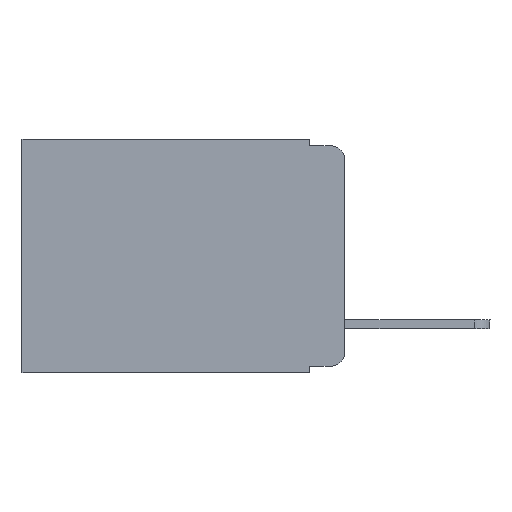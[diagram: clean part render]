
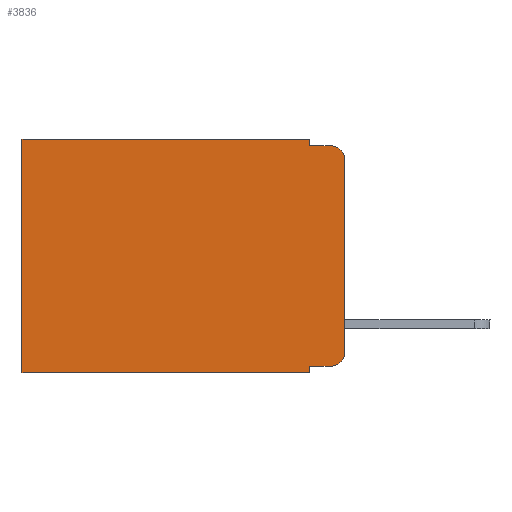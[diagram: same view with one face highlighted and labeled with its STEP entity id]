
A CAD part, left-side view. The second image highlights one B-rep face of the part: STEP entity #3836.
In plain terms, the highlighted planar face has unit normal (-1, 0, 0).
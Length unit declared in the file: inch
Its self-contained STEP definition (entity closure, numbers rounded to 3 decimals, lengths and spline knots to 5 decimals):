
#102 = CARTESIAN_POINT ( 'NONE',  ( 0.298, 0., 0. ) ) ;
#114 = DIRECTION ( 'NONE',  ( 0., 0., -1. ) ) ;
#173 = DIRECTION ( 'NONE',  ( -1., 0., 0. ) ) ;
#221 = VERTEX_POINT ( 'NONE', #9424 ) ;
#527 = ORIENTED_EDGE ( 'NONE', *, *, #11059, .T. ) ;
#671 = CARTESIAN_POINT ( 'NONE',  ( 0.298, 0.051, -0.01 ) ) ;
#741 = ORIENTED_EDGE ( 'NONE', *, *, #4557, .F. ) ;
#908 = DIRECTION ( 'NONE',  ( 0., 0., -1. ) ) ;
#916 = ORIENTED_EDGE ( 'NONE', *, *, #3849, .F. ) ;
#985 = CIRCLE ( 'NONE', #7478, 0.02 ) ;
#1032 = CARTESIAN_POINT ( 'NONE',  ( 0.298, 0.051, 0. ) ) ;
#1308 = LINE ( 'NONE', #4861, #8007 ) ;
#1367 = DIRECTION ( 'NONE',  ( 0., 1., 0. ) ) ;
#1461 = CARTESIAN_POINT ( 'NONE',  ( 0.298, 0.051, 0. ) ) ;
#1916 = VECTOR ( 'NONE', #4819, 39.37008 ) ;
#2026 = VERTEX_POINT ( 'NONE', #11433 ) ;
#2085 = EDGE_CURVE ( 'NONE', #7836, #8488, #2675, .T. ) ;
#2386 = CARTESIAN_POINT ( 'NONE',  ( 0.298, 0., 0. ) ) ;
#2560 = EDGE_CURVE ( 'NONE', #6915, #5818, #8113, .T. ) ;
#2675 = LINE ( 'NONE', #9013, #3173 ) ;
#2697 = VERTEX_POINT ( 'NONE', #1461 ) ;
#3063 = EDGE_CURVE ( 'NONE', #6915, #2026, #985, .T. ) ;
#3106 = EDGE_LOOP ( 'NONE', ( #10215, #3978, #741, #916, #527, #6102, #5213, #9577, #4777, #3183 ) ) ;
#3173 = VECTOR ( 'NONE', #4595, 39.37008 ) ;
#3183 = ORIENTED_EDGE ( 'NONE', *, *, #11185, .T. ) ;
#3337 = LINE ( 'NONE', #671, #8975 ) ;
#3636 = EDGE_CURVE ( 'NONE', #8551, #8324, #5702, .T. ) ;
#3835 = CARTESIAN_POINT ( 'NONE',  ( 0.298, 0., -0.03 ) ) ;
#3836 = ADVANCED_FACE ( 'NONE', ( #9970 ), #7310, .F. ) ;
#3849 = EDGE_CURVE ( 'NONE', #2697, #221, #7147, .T. ) ;
#3978 = ORIENTED_EDGE ( 'NONE', *, *, #3063, .T. ) ;
#4557 = EDGE_CURVE ( 'NONE', #221, #2026, #3337, .T. ) ;
#4583 = DIRECTION ( 'NONE',  ( 0., -1., 0. ) ) ;
#4595 = DIRECTION ( 'NONE',  ( 0., 0., -1. ) ) ;
#4602 = CARTESIAN_POINT ( 'NONE',  ( 0.298, 0.02, -0.333 ) ) ;
#4729 = AXIS2_PLACEMENT_3D ( 'NONE', #7092, #9015, #114 ) ;
#4777 = ORIENTED_EDGE ( 'NONE', *, *, #10180, .T. ) ;
#4819 = DIRECTION ( 'NONE',  ( 0., 0., -1. ) ) ;
#4861 = CARTESIAN_POINT ( 'NONE',  ( 0.298, 0., -0.343 ) ) ;
#5091 = CIRCLE ( 'NONE', #4729, 0.02 ) ;
#5213 = ORIENTED_EDGE ( 'NONE', *, *, #5695, .F. ) ;
#5340 = DIRECTION ( 'NONE',  ( 1., 0., 0. ) ) ;
#5647 = VECTOR ( 'NONE', #908, 39.37008 ) ;
#5695 = EDGE_CURVE ( 'NONE', #8488, #8324, #1308, .T. ) ;
#5702 = LINE ( 'NONE', #9239, #1916 ) ;
#5818 = VERTEX_POINT ( 'NONE', #7009 ) ;
#6057 = DIRECTION ( 'NONE',  ( 0., 1., 0. ) ) ;
#6102 = ORIENTED_EDGE ( 'NONE', *, *, #3636, .T. ) ;
#6137 = DIRECTION ( 'NONE',  ( 0., -1., 0. ) ) ;
#6206 = AXIS2_PLACEMENT_3D ( 'NONE', #102, #5340, #10845 ) ;
#6391 = LINE ( 'NONE', #7244, #6438 ) ;
#6438 = VECTOR ( 'NONE', #4583, 39.37008 ) ;
#6859 = CARTESIAN_POINT ( 'NONE',  ( 0.298, 0.051, -0.343 ) ) ;
#6915 = VERTEX_POINT ( 'NONE', #3835 ) ;
#7009 = CARTESIAN_POINT ( 'NONE',  ( 0.298, 0., -0.313 ) ) ;
#7092 = CARTESIAN_POINT ( 'NONE',  ( 0.298, 0.02, -0.313 ) ) ;
#7147 = LINE ( 'NONE', #1032, #5647 ) ;
#7208 = CARTESIAN_POINT ( 'NONE',  ( 0.298, 0.473, 0. ) ) ;
#7244 = CARTESIAN_POINT ( 'NONE',  ( 0.298, 0.051, -0.333 ) ) ;
#7310 = PLANE ( 'NONE',  #6206 ) ;
#7478 = AXIS2_PLACEMENT_3D ( 'NONE', #8101, #173, #10816 ) ;
#7836 = VERTEX_POINT ( 'NONE', #8376 ) ;
#8007 = VECTOR ( 'NONE', #1367, 39.37008 ) ;
#8066 = VERTEX_POINT ( 'NONE', #4602 ) ;
#8101 = CARTESIAN_POINT ( 'NONE',  ( 0.298, 0.02, -0.03 ) ) ;
#8113 = LINE ( 'NONE', #10884, #11332 ) ;
#8324 = VERTEX_POINT ( 'NONE', #10157 ) ;
#8376 = CARTESIAN_POINT ( 'NONE',  ( 0.298, 0.051, -0.333 ) ) ;
#8488 = VERTEX_POINT ( 'NONE', #6859 ) ;
#8551 = VERTEX_POINT ( 'NONE', #7208 ) ;
#8975 = VECTOR ( 'NONE', #6137, 39.37008 ) ;
#9013 = CARTESIAN_POINT ( 'NONE',  ( 0.298, 0.051, 0. ) ) ;
#9015 = DIRECTION ( 'NONE',  ( -1., 0., 0. ) ) ;
#9239 = CARTESIAN_POINT ( 'NONE',  ( 0.298, 0.473, 0. ) ) ;
#9338 = VECTOR ( 'NONE', #6057, 39.37008 ) ;
#9424 = CARTESIAN_POINT ( 'NONE',  ( 0.298, 0.051, -0.01 ) ) ;
#9577 = ORIENTED_EDGE ( 'NONE', *, *, #2085, .F. ) ;
#9970 = FACE_OUTER_BOUND ( 'NONE', #3106, .T. ) ;
#10006 = DIRECTION ( 'NONE',  ( 0., 0., -1. ) ) ;
#10157 = CARTESIAN_POINT ( 'NONE',  ( 0.298, 0.473, -0.343 ) ) ;
#10180 = EDGE_CURVE ( 'NONE', #7836, #8066, #6391, .T. ) ;
#10215 = ORIENTED_EDGE ( 'NONE', *, *, #2560, .F. ) ;
#10335 = LINE ( 'NONE', #2386, #9338 ) ;
#10816 = DIRECTION ( 'NONE',  ( 0., 0., -1. ) ) ;
#10845 = DIRECTION ( 'NONE',  ( 0., 0., -1. ) ) ;
#10884 = CARTESIAN_POINT ( 'NONE',  ( 0.298, 0., 0. ) ) ;
#11059 = EDGE_CURVE ( 'NONE', #2697, #8551, #10335, .T. ) ;
#11185 = EDGE_CURVE ( 'NONE', #8066, #5818, #5091, .T. ) ;
#11332 = VECTOR ( 'NONE', #10006, 39.37008 ) ;
#11433 = CARTESIAN_POINT ( 'NONE',  ( 0.298, 0.02, -0.01 ) ) ;
